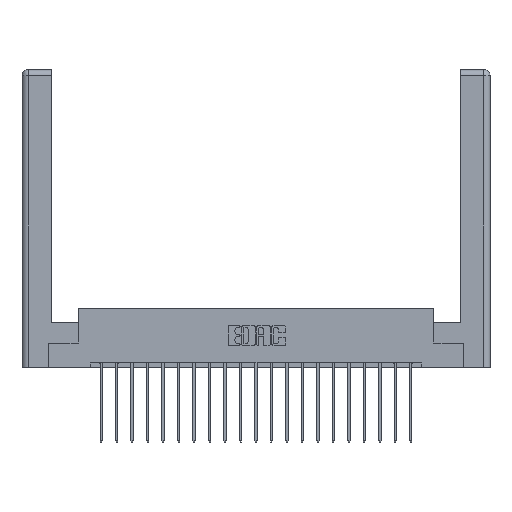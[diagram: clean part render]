
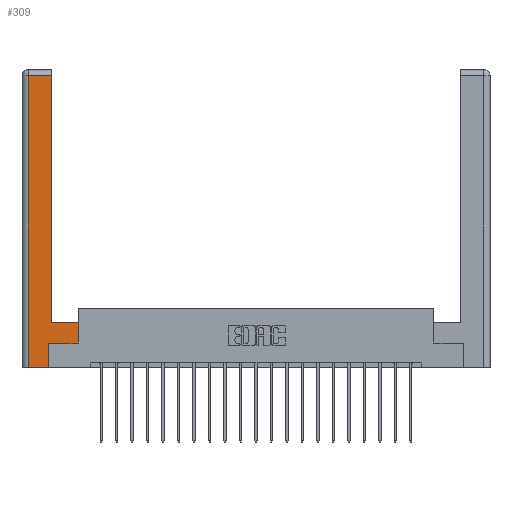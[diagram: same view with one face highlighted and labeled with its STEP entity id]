
A CAD part, top view. The second image highlights one B-rep face of the part: STEP entity #309.
In plain terms, the highlighted planar face has unit normal (0, 0, 1).
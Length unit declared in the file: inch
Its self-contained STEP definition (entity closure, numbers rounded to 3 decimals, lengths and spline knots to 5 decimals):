
#46 = CARTESIAN_POINT ( 'NONE',  ( 0.295, 0.45, 0. ) ) ;
#111 = CARTESIAN_POINT ( 'NONE',  ( 0.565, 0.45, 0. ) ) ;
#309 = ADVANCED_FACE ( 'NONE', ( #714 ), #21286, .F. ) ;
#314 = DIRECTION ( 'NONE',  ( 0., 1., 0. ) ) ;
#383 = ORIENTED_EDGE ( 'NONE', *, *, #3628, .T. ) ;
#418 = CARTESIAN_POINT ( 'NONE',  ( 0.265, 0.245, 0. ) ) ;
#449 = CARTESIAN_POINT ( 'NONE',  ( 0.0615, 2.94, 0. ) ) ;
#451 = VECTOR ( 'NONE', #19472, 39.37008 ) ;
#712 = VERTEX_POINT ( 'NONE', #4555 ) ;
#714 = FACE_OUTER_BOUND ( 'NONE', #19140, .T. ) ;
#1036 = VECTOR ( 'NONE', #5120, 39.37008 ) ;
#1204 = VECTOR ( 'NONE', #5732, 39.37008 ) ;
#1354 = EDGE_CURVE ( 'NONE', #15590, #712, #5619, .T. ) ;
#2129 = VERTEX_POINT ( 'NONE', #21667 ) ;
#2760 = DIRECTION ( 'NONE',  ( -1., 0., 0. ) ) ;
#3075 = CARTESIAN_POINT ( 'NONE',  ( 0.0615, 2.94, 0. ) ) ;
#3628 = EDGE_CURVE ( 'NONE', #2129, #4924, #5601, .T. ) ;
#4555 = CARTESIAN_POINT ( 'NONE',  ( 0.0615, 0., 0. ) ) ;
#4924 = VERTEX_POINT ( 'NONE', #13064 ) ;
#5120 = DIRECTION ( 'NONE',  ( -1., 0., 0. ) ) ;
#5254 = DIRECTION ( 'NONE',  ( 0., 1., 0. ) ) ;
#5601 = LINE ( 'NONE', #9275, #20767 ) ;
#5619 = LINE ( 'NONE', #10830, #1204 ) ;
#5732 = DIRECTION ( 'NONE',  ( 0., -1., 0. ) ) ;
#6203 = EDGE_CURVE ( 'NONE', #17977, #11776, #20278, .T. ) ;
#6209 = ORIENTED_EDGE ( 'NONE', *, *, #6660, .T. ) ;
#6634 = ORIENTED_EDGE ( 'NONE', *, *, #10449, .T. ) ;
#6660 = EDGE_CURVE ( 'NONE', #11776, #11736, #7711, .T. ) ;
#7143 = VERTEX_POINT ( 'NONE', #13226 ) ;
#7329 = CARTESIAN_POINT ( 'NONE',  ( 0.295, 3., 0. ) ) ;
#7544 = ORIENTED_EDGE ( 'NONE', *, *, #6203, .T. ) ;
#7711 = LINE ( 'NONE', #7329, #20493 ) ;
#7774 = CARTESIAN_POINT ( 'NONE',  ( 0.295, 0.45, 0. ) ) ;
#8010 = DIRECTION ( 'NONE',  ( 0., 1., 0. ) ) ;
#8017 = VECTOR ( 'NONE', #9685, 39.37008 ) ;
#8573 = CARTESIAN_POINT ( 'NONE',  ( 0.295, 2.94, 0. ) ) ;
#9275 = CARTESIAN_POINT ( 'NONE',  ( 0.565, 0.245, 0. ) ) ;
#9560 = CARTESIAN_POINT ( 'NONE',  ( 0.265, 0., 0. ) ) ;
#9685 = DIRECTION ( 'NONE',  ( -1., 0., 0. ) ) ;
#9752 = CARTESIAN_POINT ( 'NONE',  ( 0., 0., 0. ) ) ;
#10449 = EDGE_CURVE ( 'NONE', #712, #7143, #15595, .T. ) ;
#10830 = CARTESIAN_POINT ( 'NONE',  ( 0.0615, 0., 0. ) ) ;
#11297 = ORIENTED_EDGE ( 'NONE', *, *, #1354, .T. ) ;
#11379 = EDGE_CURVE ( 'NONE', #4924, #17977, #14165, .T. ) ;
#11413 = LINE ( 'NONE', #418, #13248 ) ;
#11736 = VERTEX_POINT ( 'NONE', #8573 ) ;
#11776 = VERTEX_POINT ( 'NONE', #46 ) ;
#12084 = EDGE_CURVE ( 'NONE', #11736, #15590, #14927, .T. ) ;
#13064 = CARTESIAN_POINT ( 'NONE',  ( 0.565, 0.245, 0. ) ) ;
#13226 = CARTESIAN_POINT ( 'NONE',  ( 0.265, 0., 0. ) ) ;
#13248 = VECTOR ( 'NONE', #5254, 39.37008 ) ;
#14165 = LINE ( 'NONE', #18022, #19356 ) ;
#14405 = DIRECTION ( 'NONE',  ( 1., 0., 0. ) ) ;
#14461 = ORIENTED_EDGE ( 'NONE', *, *, #11379, .T. ) ;
#14927 = LINE ( 'NONE', #3075, #1036 ) ;
#15590 = VERTEX_POINT ( 'NONE', #449 ) ;
#15595 = LINE ( 'NONE', #9560, #451 ) ;
#16649 = ORIENTED_EDGE ( 'NONE', *, *, #20930, .T. ) ;
#17302 = AXIS2_PLACEMENT_3D ( 'NONE', #9752, #19744, #2760 ) ;
#17977 = VERTEX_POINT ( 'NONE', #111 ) ;
#18022 = CARTESIAN_POINT ( 'NONE',  ( 0.565, 0.45, 0. ) ) ;
#18543 = ORIENTED_EDGE ( 'NONE', *, *, #12084, .T. ) ;
#19140 = EDGE_LOOP ( 'NONE', ( #6209, #18543, #11297, #6634, #16649, #383, #14461, #7544 ) ) ;
#19356 = VECTOR ( 'NONE', #8010, 39.37008 ) ;
#19472 = DIRECTION ( 'NONE',  ( 1., 0., 0. ) ) ;
#19744 = DIRECTION ( 'NONE',  ( 0., 0., -1. ) ) ;
#20278 = LINE ( 'NONE', #7774, #8017 ) ;
#20493 = VECTOR ( 'NONE', #314, 39.37008 ) ;
#20767 = VECTOR ( 'NONE', #14405, 39.37008 ) ;
#20930 = EDGE_CURVE ( 'NONE', #7143, #2129, #11413, .T. ) ;
#21286 = PLANE ( 'NONE',  #17302 ) ;
#21667 = CARTESIAN_POINT ( 'NONE',  ( 0.265, 0.245, 0. ) ) ;
